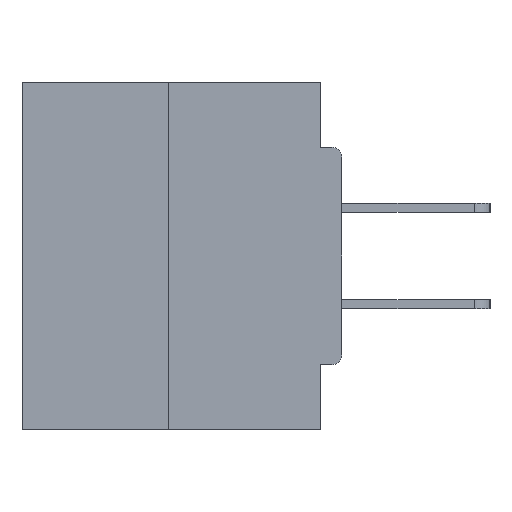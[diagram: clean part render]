
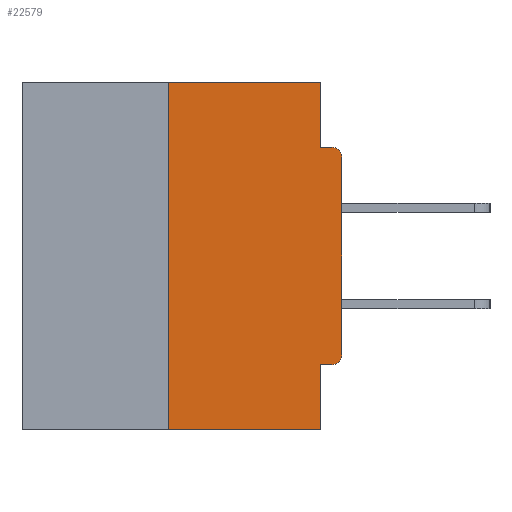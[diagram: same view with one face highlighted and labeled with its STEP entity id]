
A CAD part, left-side view. The second image highlights one B-rep face of the part: STEP entity #22579.
In plain terms, the highlighted planar face has unit normal (-1, 0, 0).
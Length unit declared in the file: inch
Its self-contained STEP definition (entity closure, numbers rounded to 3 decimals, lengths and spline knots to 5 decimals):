
#28 = VERTEX_POINT ( 'NONE', #10115 ) ;
#271 = CIRCLE ( 'NONE', #6831, 0.015 ) ;
#455 = CARTESIAN_POINT ( 'NONE',  ( 0., 0.25, 0. ) ) ;
#586 = LINE ( 'NONE', #16738, #10185 ) ;
#624 = LINE ( 'NONE', #15821, #3723 ) ;
#1088 = VECTOR ( 'NONE', #33712, 39.37008 ) ;
#1664 = DIRECTION ( 'NONE',  ( 0., 0., -1. ) ) ;
#3723 = VECTOR ( 'NONE', #32539, 39.37008 ) ;
#3991 = DIRECTION ( 'NONE',  ( 0., 0., -1. ) ) ;
#4147 = VECTOR ( 'NONE', #26970, 39.37008 ) ;
#4642 = VERTEX_POINT ( 'NONE', #32341 ) ;
#5329 = ORIENTED_EDGE ( 'NONE', *, *, #17129, .F. ) ;
#6024 = ORIENTED_EDGE ( 'NONE', *, *, #30341, .T. ) ;
#6060 = CARTESIAN_POINT ( 'NONE',  ( 0., 0., -0.3915 ) ) ;
#6831 = AXIS2_PLACEMENT_3D ( 'NONE', #24901, #30922, #22112 ) ;
#7341 = FACE_OUTER_BOUND ( 'NONE', #20970, .T. ) ;
#7708 = VERTEX_POINT ( 'NONE', #9526 ) ;
#7740 = VECTOR ( 'NONE', #26977, 39.37008 ) ;
#8078 = VERTEX_POINT ( 'NONE', #455 ) ;
#8243 = DIRECTION ( 'NONE',  ( 0., -1., 0. ) ) ;
#8700 = CARTESIAN_POINT ( 'NONE',  ( 0., 0., -0.1085 ) ) ;
#8910 = ORIENTED_EDGE ( 'NONE', *, *, #15175, .T. ) ;
#9315 = CIRCLE ( 'NONE', #28065, 0.015 ) ;
#9526 = CARTESIAN_POINT ( 'NONE',  ( 0., 0.015, -0.4065 ) ) ;
#9686 = PLANE ( 'NONE',  #17056 ) ;
#9967 = CARTESIAN_POINT ( 'NONE',  ( 0., 0.015, -0.1085 ) ) ;
#10115 = CARTESIAN_POINT ( 'NONE',  ( 0., 0.031, 0. ) ) ;
#10185 = VECTOR ( 'NONE', #8243, 39.37008 ) ;
#10742 = VERTEX_POINT ( 'NONE', #8700 ) ;
#11390 = DIRECTION ( 'NONE',  ( 0., 0., 1. ) ) ;
#11979 = CARTESIAN_POINT ( 'NONE',  ( 0., 0.031, -0.0935 ) ) ;
#13224 = LINE ( 'NONE', #34855, #4147 ) ;
#13262 = LINE ( 'NONE', #34938, #30162 ) ;
#13357 = ORIENTED_EDGE ( 'NONE', *, *, #18522, .F. ) ;
#15175 = EDGE_CURVE ( 'NONE', #22401, #18271, #586, .T. ) ;
#15498 = EDGE_CURVE ( 'NONE', #26729, #10742, #33589, .T. ) ;
#15821 = CARTESIAN_POINT ( 'NONE',  ( 0., 0.25, 0. ) ) ;
#15923 = ORIENTED_EDGE ( 'NONE', *, *, #31434, .F. ) ;
#16612 = VERTEX_POINT ( 'NONE', #21826 ) ;
#16738 = CARTESIAN_POINT ( 'NONE',  ( 0., 0.46, -0.5 ) ) ;
#17056 = AXIS2_PLACEMENT_3D ( 'NONE', #23418, #29072, #3991 ) ;
#17129 = EDGE_CURVE ( 'NONE', #28, #29107, #31152, .T. ) ;
#17936 = ORIENTED_EDGE ( 'NONE', *, *, #15498, .T. ) ;
#18197 = DIRECTION ( 'NONE',  ( -1., 0., 0. ) ) ;
#18271 = VERTEX_POINT ( 'NONE', #20595 ) ;
#18380 = EDGE_CURVE ( 'NONE', #29107, #16612, #13262, .T. ) ;
#18522 = EDGE_CURVE ( 'NONE', #7708, #4642, #23302, .T. ) ;
#18637 = EDGE_CURVE ( 'NONE', #4642, #18271, #13224, .T. ) ;
#19080 = DIRECTION ( 'NONE',  ( 0., -1., 0. ) ) ;
#19652 = CARTESIAN_POINT ( 'NONE',  ( 0., 0., 0. ) ) ;
#20595 = CARTESIAN_POINT ( 'NONE',  ( 0., 0.031, -0.5 ) ) ;
#20970 = EDGE_LOOP ( 'NONE', ( #22923, #15923, #8910, #21476, #13357, #6024, #17936, #33260, #35046, #5329 ) ) ;
#21476 = ORIENTED_EDGE ( 'NONE', *, *, #18637, .F. ) ;
#21826 = CARTESIAN_POINT ( 'NONE',  ( 0., 0.015, -0.0935 ) ) ;
#22112 = DIRECTION ( 'NONE',  ( 0., 0., -1. ) ) ;
#22401 = VERTEX_POINT ( 'NONE', #32268 ) ;
#22579 = ADVANCED_FACE ( 'NONE', ( #7341 ), #9686, .F. ) ;
#22923 = ORIENTED_EDGE ( 'NONE', *, *, #23442, .F. ) ;
#23302 = LINE ( 'NONE', #25599, #1088 ) ;
#23418 = CARTESIAN_POINT ( 'NONE',  ( 0., 0.46, 0. ) ) ;
#23442 = EDGE_CURVE ( 'NONE', #8078, #28, #31562, .T. ) ;
#23587 = DIRECTION ( 'NONE',  ( 0., -1., 0. ) ) ;
#24901 = CARTESIAN_POINT ( 'NONE',  ( 0., 0.015, -0.3915 ) ) ;
#24915 = CARTESIAN_POINT ( 'NONE',  ( 0., 0.46, 0. ) ) ;
#25189 = EDGE_CURVE ( 'NONE', #10742, #16612, #9315, .T. ) ;
#25533 = VECTOR ( 'NONE', #19080, 39.37008 ) ;
#25599 = CARTESIAN_POINT ( 'NONE',  ( 0., 0., -0.4065 ) ) ;
#25777 = VECTOR ( 'NONE', #11390, 39.37008 ) ;
#26729 = VERTEX_POINT ( 'NONE', #6060 ) ;
#26970 = DIRECTION ( 'NONE',  ( 0., 0., -1. ) ) ;
#26977 = DIRECTION ( 'NONE',  ( 0., 0., -1. ) ) ;
#28065 = AXIS2_PLACEMENT_3D ( 'NONE', #9967, #18197, #1664 ) ;
#29072 = DIRECTION ( 'NONE',  ( 1., 0., 0. ) ) ;
#29107 = VERTEX_POINT ( 'NONE', #11979 ) ;
#30162 = VECTOR ( 'NONE', #23587, 39.37008 ) ;
#30341 = EDGE_CURVE ( 'NONE', #7708, #26729, #271, .T. ) ;
#30922 = DIRECTION ( 'NONE',  ( -1., 0., 0. ) ) ;
#31152 = LINE ( 'NONE', #32297, #7740 ) ;
#31434 = EDGE_CURVE ( 'NONE', #22401, #8078, #624, .T. ) ;
#31562 = LINE ( 'NONE', #24915, #25533 ) ;
#32268 = CARTESIAN_POINT ( 'NONE',  ( 0., 0.25, -0.5 ) ) ;
#32297 = CARTESIAN_POINT ( 'NONE',  ( 0., 0.031, 0. ) ) ;
#32341 = CARTESIAN_POINT ( 'NONE',  ( 0., 0.031, -0.4065 ) ) ;
#32539 = DIRECTION ( 'NONE',  ( 0., 0., 1. ) ) ;
#33260 = ORIENTED_EDGE ( 'NONE', *, *, #25189, .T. ) ;
#33589 = LINE ( 'NONE', #19652, #25777 ) ;
#33712 = DIRECTION ( 'NONE',  ( 0., 1., 0. ) ) ;
#34855 = CARTESIAN_POINT ( 'NONE',  ( 0., 0.031, -0.5 ) ) ;
#34938 = CARTESIAN_POINT ( 'NONE',  ( 0., 0., -0.0935 ) ) ;
#35046 = ORIENTED_EDGE ( 'NONE', *, *, #18380, .F. ) ;
